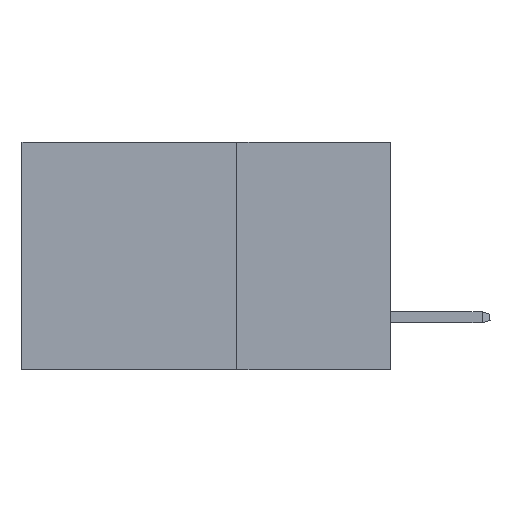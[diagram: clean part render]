
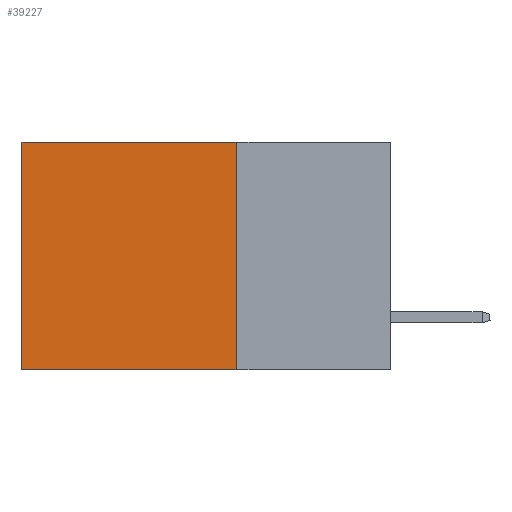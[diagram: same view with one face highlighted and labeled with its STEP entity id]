
A CAD part, left-side view. The second image highlights one B-rep face of the part: STEP entity #39227.
In plain terms, the highlighted planar face has unit normal (-1, 0, 0).
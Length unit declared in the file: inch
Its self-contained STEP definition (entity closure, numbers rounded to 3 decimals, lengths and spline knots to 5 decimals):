
#1127 = CARTESIAN_POINT ( 'NONE',  ( 0.2875, 0.25, 0. ) ) ;
#2060 = VECTOR ( 'NONE', #6296, 39.37008 ) ;
#4023 = LINE ( 'NONE', #16483, #39578 ) ;
#6262 = EDGE_CURVE ( 'NONE', #19787, #43638, #4023, .T. ) ;
#6296 = DIRECTION ( 'NONE',  ( 0., 1., 0. ) ) ;
#6498 = VERTEX_POINT ( 'NONE', #18329 ) ;
#8489 = DIRECTION ( 'NONE',  ( 1., 0., 0. ) ) ;
#9075 = DIRECTION ( 'NONE',  ( 0., 0., -1. ) ) ;
#9095 = CARTESIAN_POINT ( 'NONE',  ( 0.2875, 0.25, -0.37 ) ) ;
#9833 = DIRECTION ( 'NONE',  ( 0., 0., -1. ) ) ;
#11870 = LINE ( 'NONE', #29514, #16778 ) ;
#11931 = EDGE_LOOP ( 'NONE', ( #30608, #30962, #28052, #18970 ) ) ;
#15130 = EDGE_CURVE ( 'NONE', #6498, #42208, #11870, .T. ) ;
#16483 = CARTESIAN_POINT ( 'NONE',  ( 0.2875, 0.25, 0. ) ) ;
#16778 = VECTOR ( 'NONE', #9075, 39.37008 ) ;
#18329 = CARTESIAN_POINT ( 'NONE',  ( 0.2875, 0.6, 0. ) ) ;
#18970 = ORIENTED_EDGE ( 'NONE', *, *, #38806, .T. ) ;
#19787 = VERTEX_POINT ( 'NONE', #1127 ) ;
#19998 = CARTESIAN_POINT ( 'NONE',  ( 0.2875, 0.25, 0. ) ) ;
#21569 = CARTESIAN_POINT ( 'NONE',  ( 0.2875, 0.25, -0.37 ) ) ;
#22376 = LINE ( 'NONE', #21569, #30414 ) ;
#23772 = AXIS2_PLACEMENT_3D ( 'NONE', #39338, #8489, #25192 ) ;
#25192 = DIRECTION ( 'NONE',  ( 0., 0., -1. ) ) ;
#26432 = EDGE_CURVE ( 'NONE', #43638, #42208, #22376, .T. ) ;
#28052 = ORIENTED_EDGE ( 'NONE', *, *, #6262, .F. ) ;
#29078 = CARTESIAN_POINT ( 'NONE',  ( 0.2875, 0.6, -0.37 ) ) ;
#29514 = CARTESIAN_POINT ( 'NONE',  ( 0.2875, 0.6, 0. ) ) ;
#29989 = LINE ( 'NONE', #19998, #2060 ) ;
#30414 = VECTOR ( 'NONE', #35408, 39.37008 ) ;
#30608 = ORIENTED_EDGE ( 'NONE', *, *, #15130, .T. ) ;
#30962 = ORIENTED_EDGE ( 'NONE', *, *, #26432, .F. ) ;
#32087 = PLANE ( 'NONE',  #23772 ) ;
#34262 = FACE_OUTER_BOUND ( 'NONE', #11931, .T. ) ;
#35408 = DIRECTION ( 'NONE',  ( 0., 1., 0. ) ) ;
#38806 = EDGE_CURVE ( 'NONE', #19787, #6498, #29989, .T. ) ;
#39227 = ADVANCED_FACE ( 'NONE', ( #34262 ), #32087, .F. ) ;
#39338 = CARTESIAN_POINT ( 'NONE',  ( 0.2875, 0.25, 0. ) ) ;
#39578 = VECTOR ( 'NONE', #9833, 39.37008 ) ;
#42208 = VERTEX_POINT ( 'NONE', #29078 ) ;
#43638 = VERTEX_POINT ( 'NONE', #9095 ) ;
